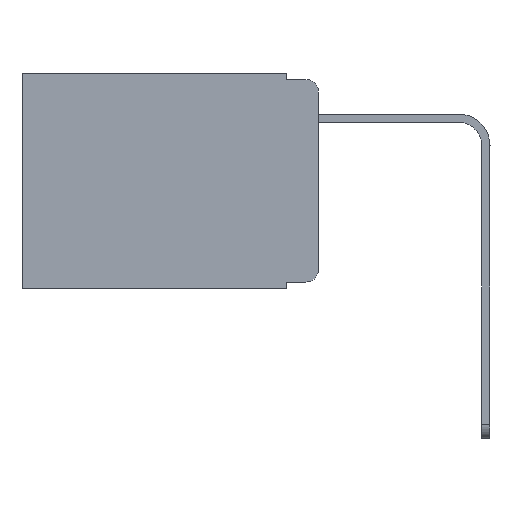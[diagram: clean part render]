
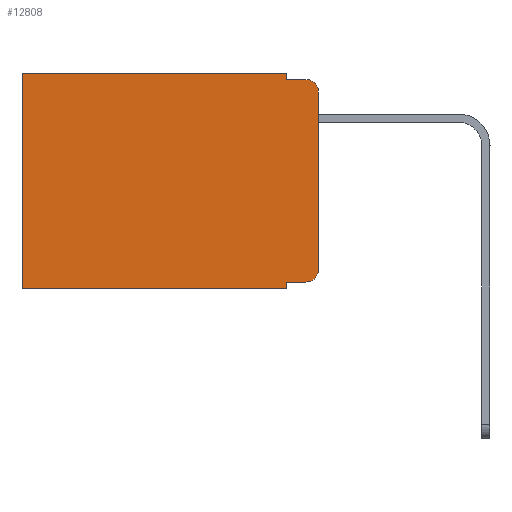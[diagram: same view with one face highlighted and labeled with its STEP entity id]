
A CAD part, left-side view. The second image highlights one B-rep face of the part: STEP entity #12808.
In plain terms, the highlighted planar face has unit normal (-1, 0, 0).
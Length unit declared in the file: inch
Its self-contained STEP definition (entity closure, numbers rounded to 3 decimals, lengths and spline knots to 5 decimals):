
#282 = ORIENTED_EDGE ( 'NONE', *, *, #8351, .T. ) ;
#338 = EDGE_CURVE ( 'NONE', #9353, #11825, #10759, .T. ) ;
#471 = ORIENTED_EDGE ( 'NONE', *, *, #7634, .F. ) ;
#560 = ORIENTED_EDGE ( 'NONE', *, *, #12548, .T. ) ;
#720 = VECTOR ( 'NONE', #3821, 39.37008 ) ;
#766 = VECTOR ( 'NONE', #5626, 39.37008 ) ;
#929 = CARTESIAN_POINT ( 'NONE',  ( 0.298, 0.051, -0.333 ) ) ;
#942 = LINE ( 'NONE', #5715, #766 ) ;
#1007 = CARTESIAN_POINT ( 'NONE',  ( 0.298, 0.473, -0.343 ) ) ;
#1010 = EDGE_CURVE ( 'NONE', #7996, #8670, #8057, .T. ) ;
#1069 = CIRCLE ( 'NONE', #13125, 0.02 ) ;
#1422 = EDGE_CURVE ( 'NONE', #3838, #8670, #7400, .T. ) ;
#1615 = ORIENTED_EDGE ( 'NONE', *, *, #9753, .F. ) ;
#2160 = VERTEX_POINT ( 'NONE', #2804 ) ;
#2349 = CARTESIAN_POINT ( 'NONE',  ( 0.298, 0.051, 0. ) ) ;
#2415 = LINE ( 'NONE', #4667, #3564 ) ;
#2425 = VECTOR ( 'NONE', #7450, 39.37008 ) ;
#2625 = PLANE ( 'NONE',  #6974 ) ;
#2804 = CARTESIAN_POINT ( 'NONE',  ( 0.298, 0.051, -0.333 ) ) ;
#2866 = DIRECTION ( 'NONE',  ( 0., -1., 0. ) ) ;
#2971 = DIRECTION ( 'NONE',  ( -1., 0., 0. ) ) ;
#3118 = DIRECTION ( 'NONE',  ( 0., 0., -1. ) ) ;
#3564 = VECTOR ( 'NONE', #13079, 39.37008 ) ;
#3697 = DIRECTION ( 'NONE',  ( 1., 0., 0. ) ) ;
#3821 = DIRECTION ( 'NONE',  ( 0., 1., 0. ) ) ;
#3838 = VERTEX_POINT ( 'NONE', #13203 ) ;
#4068 = VERTEX_POINT ( 'NONE', #8820 ) ;
#4660 = EDGE_CURVE ( 'NONE', #2160, #3838, #10814, .T. ) ;
#4667 = CARTESIAN_POINT ( 'NONE',  ( 0.298, 0., 0. ) ) ;
#5161 = DIRECTION ( 'NONE',  ( -1., 0., 0. ) ) ;
#5223 = VECTOR ( 'NONE', #7843, 39.37008 ) ;
#5579 = EDGE_CURVE ( 'NONE', #6209, #7009, #1069, .T. ) ;
#5626 = DIRECTION ( 'NONE',  ( 0., 0., -1. ) ) ;
#5715 = CARTESIAN_POINT ( 'NONE',  ( 0.298, 0.051, 0. ) ) ;
#5732 = DIRECTION ( 'NONE',  ( 0., 0., -1. ) ) ;
#6209 = VERTEX_POINT ( 'NONE', #10052 ) ;
#6375 = DIRECTION ( 'NONE',  ( 0., 0., -1. ) ) ;
#6666 = EDGE_LOOP ( 'NONE', ( #471, #8928, #11834, #1615, #282, #13492, #7818, #12006, #560, #10719 ) ) ;
#6898 = CARTESIAN_POINT ( 'NONE',  ( 0.298, 0., 0. ) ) ;
#6953 = LINE ( 'NONE', #929, #2425 ) ;
#6974 = AXIS2_PLACEMENT_3D ( 'NONE', #6898, #3697, #5732 ) ;
#7009 = VERTEX_POINT ( 'NONE', #12192 ) ;
#7267 = DIRECTION ( 'NONE',  ( 0., 0., -1. ) ) ;
#7274 = FACE_OUTER_BOUND ( 'NONE', #6666, .T. ) ;
#7400 = LINE ( 'NONE', #12309, #720 ) ;
#7450 = DIRECTION ( 'NONE',  ( 0., -1., 0. ) ) ;
#7634 = EDGE_CURVE ( 'NONE', #4068, #7009, #9892, .T. ) ;
#7818 = ORIENTED_EDGE ( 'NONE', *, *, #1422, .F. ) ;
#7843 = DIRECTION ( 'NONE',  ( 0., 0., -1. ) ) ;
#7996 = VERTEX_POINT ( 'NONE', #9845 ) ;
#8057 = LINE ( 'NONE', #8294, #12571 ) ;
#8294 = CARTESIAN_POINT ( 'NONE',  ( 0.298, 0.473, 0. ) ) ;
#8351 = EDGE_CURVE ( 'NONE', #13389, #7996, #2415, .T. ) ;
#8629 = VECTOR ( 'NONE', #6375, 39.37008 ) ;
#8670 = VERTEX_POINT ( 'NONE', #1007 ) ;
#8820 = CARTESIAN_POINT ( 'NONE',  ( 0.298, 0., -0.03 ) ) ;
#8928 = ORIENTED_EDGE ( 'NONE', *, *, #10690, .T. ) ;
#9353 = VERTEX_POINT ( 'NONE', #9362 ) ;
#9362 = CARTESIAN_POINT ( 'NONE',  ( 0.298, 0.051, -0.01 ) ) ;
#9753 = EDGE_CURVE ( 'NONE', #13389, #9353, #942, .T. ) ;
#9845 = CARTESIAN_POINT ( 'NONE',  ( 0.298, 0.473, 0. ) ) ;
#9892 = LINE ( 'NONE', #11188, #5223 ) ;
#10052 = CARTESIAN_POINT ( 'NONE',  ( 0.298, 0.02, -0.333 ) ) ;
#10090 = VECTOR ( 'NONE', #2866, 39.37008 ) ;
#10301 = CARTESIAN_POINT ( 'NONE',  ( 0.298, 0.02, -0.01 ) ) ;
#10512 = CARTESIAN_POINT ( 'NONE',  ( 0.298, 0.051, -0.01 ) ) ;
#10690 = EDGE_CURVE ( 'NONE', #4068, #11825, #13729, .T. ) ;
#10719 = ORIENTED_EDGE ( 'NONE', *, *, #5579, .T. ) ;
#10759 = LINE ( 'NONE', #10512, #10090 ) ;
#10814 = LINE ( 'NONE', #2349, #8629 ) ;
#11188 = CARTESIAN_POINT ( 'NONE',  ( 0.298, 0., 0. ) ) ;
#11542 = DIRECTION ( 'NONE',  ( 0., 0., -1. ) ) ;
#11825 = VERTEX_POINT ( 'NONE', #10301 ) ;
#11834 = ORIENTED_EDGE ( 'NONE', *, *, #338, .F. ) ;
#12006 = ORIENTED_EDGE ( 'NONE', *, *, #4660, .F. ) ;
#12192 = CARTESIAN_POINT ( 'NONE',  ( 0.298, 0., -0.313 ) ) ;
#12309 = CARTESIAN_POINT ( 'NONE',  ( 0.298, 0., -0.343 ) ) ;
#12548 = EDGE_CURVE ( 'NONE', #2160, #6209, #6953, .T. ) ;
#12571 = VECTOR ( 'NONE', #7267, 39.37008 ) ;
#12616 = CARTESIAN_POINT ( 'NONE',  ( 0.298, 0.02, -0.03 ) ) ;
#12664 = AXIS2_PLACEMENT_3D ( 'NONE', #12616, #5161, #3118 ) ;
#12788 = CARTESIAN_POINT ( 'NONE',  ( 0.298, 0.051, 0. ) ) ;
#12808 = ADVANCED_FACE ( 'NONE', ( #7274 ), #2625, .F. ) ;
#13079 = DIRECTION ( 'NONE',  ( 0., 1., 0. ) ) ;
#13125 = AXIS2_PLACEMENT_3D ( 'NONE', #13542, #2971, #11542 ) ;
#13203 = CARTESIAN_POINT ( 'NONE',  ( 0.298, 0.051, -0.343 ) ) ;
#13389 = VERTEX_POINT ( 'NONE', #12788 ) ;
#13492 = ORIENTED_EDGE ( 'NONE', *, *, #1010, .T. ) ;
#13542 = CARTESIAN_POINT ( 'NONE',  ( 0.298, 0.02, -0.313 ) ) ;
#13729 = CIRCLE ( 'NONE', #12664, 0.02 ) ;
